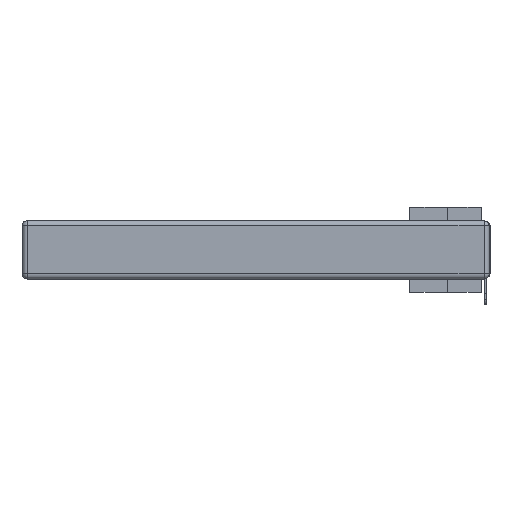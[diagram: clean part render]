
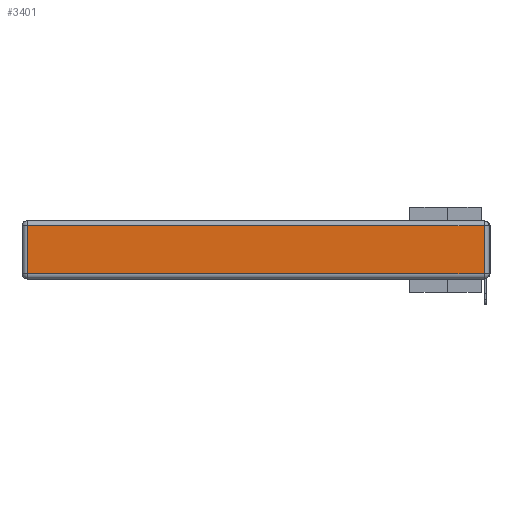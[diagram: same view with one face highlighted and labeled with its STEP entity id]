
A CAD part, left-side view. The second image highlights one B-rep face of the part: STEP entity #3401.
In plain terms, the highlighted planar face has unit normal (-1, 0, 0).
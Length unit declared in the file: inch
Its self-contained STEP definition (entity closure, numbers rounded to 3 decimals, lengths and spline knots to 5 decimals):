
#35 = VECTOR ( 'NONE', #8538, 39.37008 ) ;
#218 = ORIENTED_EDGE ( 'NONE', *, *, #25809, .T. ) ;
#1460 = LINE ( 'NONE', #33420, #7098 ) ;
#1770 = LINE ( 'NONE', #33590, #35 ) ;
#3401 = ADVANCED_FACE ( 'NONE', ( #17565 ), #26985, .T. ) ;
#4176 = DIRECTION ( 'NONE',  ( 0., 0., 1. ) ) ;
#4410 = CARTESIAN_POINT ( 'NONE',  ( 0., 0.03, -0.343 ) ) ;
#7098 = VECTOR ( 'NONE', #16559, 39.37008 ) ;
#7651 = CARTESIAN_POINT ( 'NONE',  ( 0., 0., -0.343 ) ) ;
#8538 = DIRECTION ( 'NONE',  ( 0., 1., 0. ) ) ;
#10000 = CARTESIAN_POINT ( 'NONE',  ( 0., 2.72, -0.313 ) ) ;
#11727 = VERTEX_POINT ( 'NONE', #10000 ) ;
#12209 = CARTESIAN_POINT ( 'NONE',  ( 0., 0.03, -0.03 ) ) ;
#14394 = EDGE_LOOP ( 'NONE', ( #29331, #17283, #16477, #218 ) ) ;
#14407 = AXIS2_PLACEMENT_3D ( 'NONE', #7651, #18820, #35124 ) ;
#16477 = ORIENTED_EDGE ( 'NONE', *, *, #20752, .T. ) ;
#16559 = DIRECTION ( 'NONE',  ( 0., 0., -1. ) ) ;
#16952 = CARTESIAN_POINT ( 'NONE',  ( 0., 0., -0.313 ) ) ;
#17013 = LINE ( 'NONE', #4410, #26158 ) ;
#17283 = ORIENTED_EDGE ( 'NONE', *, *, #20417, .T. ) ;
#17565 = FACE_OUTER_BOUND ( 'NONE', #14394, .T. ) ;
#17754 = EDGE_CURVE ( 'NONE', #11727, #17920, #33248, .T. ) ;
#17920 = VERTEX_POINT ( 'NONE', #29504 ) ;
#18820 = DIRECTION ( 'NONE',  ( -1., 0., 0. ) ) ;
#20417 = EDGE_CURVE ( 'NONE', #17920, #32433, #17013, .T. ) ;
#20752 = EDGE_CURVE ( 'NONE', #32433, #33845, #1770, .T. ) ;
#25809 = EDGE_CURVE ( 'NONE', #33845, #11727, #1460, .T. ) ;
#26158 = VECTOR ( 'NONE', #4176, 39.37008 ) ;
#26328 = CARTESIAN_POINT ( 'NONE',  ( 0., 2.72, -0.03 ) ) ;
#26985 = PLANE ( 'NONE',  #14407 ) ;
#29331 = ORIENTED_EDGE ( 'NONE', *, *, #17754, .T. ) ;
#29504 = CARTESIAN_POINT ( 'NONE',  ( 0., 0.03, -0.313 ) ) ;
#32433 = VERTEX_POINT ( 'NONE', #12209 ) ;
#33248 = LINE ( 'NONE', #16952, #33673 ) ;
#33420 = CARTESIAN_POINT ( 'NONE',  ( 0., 2.72, -0.343 ) ) ;
#33503 = DIRECTION ( 'NONE',  ( 0., -1., 0. ) ) ;
#33590 = CARTESIAN_POINT ( 'NONE',  ( 0., 2.75, -0.03 ) ) ;
#33673 = VECTOR ( 'NONE', #33503, 39.37008 ) ;
#33845 = VERTEX_POINT ( 'NONE', #26328 ) ;
#35124 = DIRECTION ( 'NONE',  ( 0., 0., 1. ) ) ;
